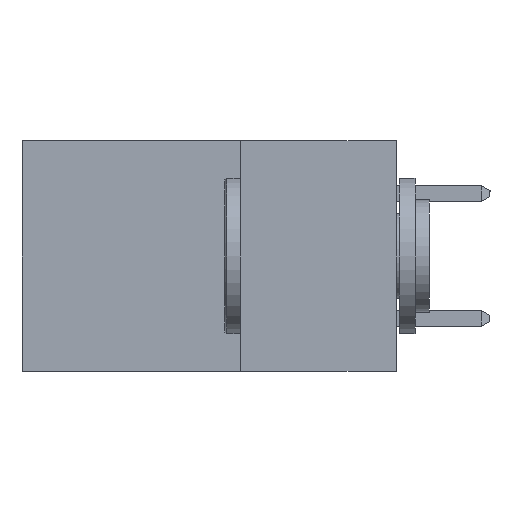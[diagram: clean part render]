
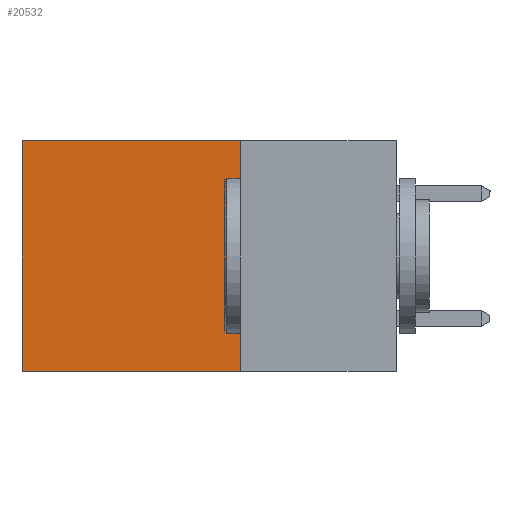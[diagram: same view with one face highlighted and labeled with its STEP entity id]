
A CAD part, left-side view. The second image highlights one B-rep face of the part: STEP entity #20532.
In plain terms, the highlighted planar face has unit normal (-1, 0, 0).
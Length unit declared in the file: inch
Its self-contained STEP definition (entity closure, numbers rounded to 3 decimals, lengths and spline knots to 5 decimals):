
#216 = EDGE_LOOP ( 'NONE', ( #13050, #17286, #19069, #21777 ) ) ;
#226 = DIRECTION ( 'NONE',  ( 0., 1., 0. ) ) ;
#321 = CARTESIAN_POINT ( 'NONE',  ( 0.2615, 0.6, 0. ) ) ;
#1300 = DIRECTION ( 'NONE',  ( 1., 0., 0. ) ) ;
#1684 = LINE ( 'NONE', #15096, #17762 ) ;
#1691 = LINE ( 'NONE', #12083, #9609 ) ;
#2554 = AXIS2_PLACEMENT_3D ( 'NONE', #20184, #1300, #13162 ) ;
#4161 = CARTESIAN_POINT ( 'NONE',  ( 0.2615, 0.6, -0.37 ) ) ;
#5028 = VECTOR ( 'NONE', #19568, 39.37008 ) ;
#6083 = CARTESIAN_POINT ( 'NONE',  ( 0.2615, 0.25, 0. ) ) ;
#6373 = VERTEX_POINT ( 'NONE', #321 ) ;
#8668 = CARTESIAN_POINT ( 'NONE',  ( 0.2615, 0.25, -0.37 ) ) ;
#9428 = VERTEX_POINT ( 'NONE', #4161 ) ;
#9609 = VECTOR ( 'NONE', #226, 39.37008 ) ;
#10338 = VECTOR ( 'NONE', #11224, 39.37008 ) ;
#11224 = DIRECTION ( 'NONE',  ( 0., 1., 0. ) ) ;
#11261 = EDGE_CURVE ( 'NONE', #6373, #9428, #1684, .T. ) ;
#11823 = VERTEX_POINT ( 'NONE', #14730 ) ;
#12083 = CARTESIAN_POINT ( 'NONE',  ( 0.2615, 0.25, -0.37 ) ) ;
#13050 = ORIENTED_EDGE ( 'NONE', *, *, #11261, .T. ) ;
#13162 = DIRECTION ( 'NONE',  ( 0., 0., -1. ) ) ;
#14730 = CARTESIAN_POINT ( 'NONE',  ( 0.2615, 0.25, 0. ) ) ;
#15096 = CARTESIAN_POINT ( 'NONE',  ( 0.2615, 0.6, -0.37 ) ) ;
#15488 = VERTEX_POINT ( 'NONE', #8668 ) ;
#15860 = EDGE_CURVE ( 'NONE', #11823, #6373, #21389, .T. ) ;
#16328 = LINE ( 'NONE', #19448, #5028 ) ;
#16608 = PLANE ( 'NONE',  #2554 ) ;
#16848 = EDGE_CURVE ( 'NONE', #11823, #15488, #16328, .T. ) ;
#17133 = EDGE_CURVE ( 'NONE', #15488, #9428, #1691, .T. ) ;
#17286 = ORIENTED_EDGE ( 'NONE', *, *, #17133, .F. ) ;
#17762 = VECTOR ( 'NONE', #18336, 39.37008 ) ;
#18182 = FACE_OUTER_BOUND ( 'NONE', #216, .T. ) ;
#18336 = DIRECTION ( 'NONE',  ( 0., 0., -1. ) ) ;
#19069 = ORIENTED_EDGE ( 'NONE', *, *, #16848, .F. ) ;
#19448 = CARTESIAN_POINT ( 'NONE',  ( 0.2615, 0.25, -0.37 ) ) ;
#19568 = DIRECTION ( 'NONE',  ( 0., 0., -1. ) ) ;
#20184 = CARTESIAN_POINT ( 'NONE',  ( 0.2615, 0.25, -0.37 ) ) ;
#20532 = ADVANCED_FACE ( 'NONE', ( #18182 ), #16608, .F. ) ;
#21389 = LINE ( 'NONE', #6083, #10338 ) ;
#21777 = ORIENTED_EDGE ( 'NONE', *, *, #15860, .T. ) ;
